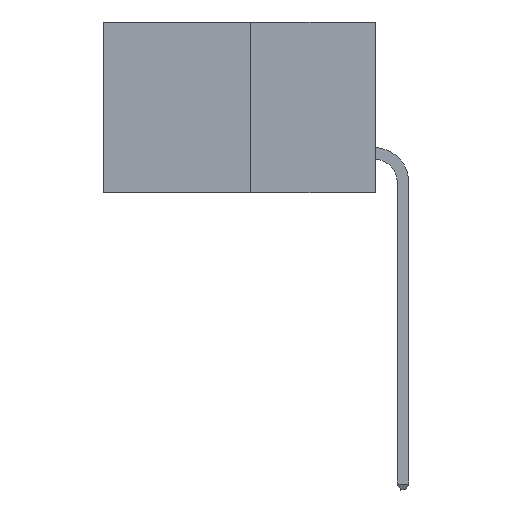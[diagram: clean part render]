
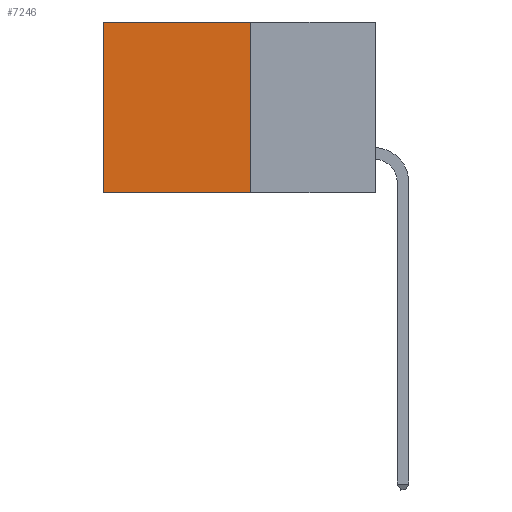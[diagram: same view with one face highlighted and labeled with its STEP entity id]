
A CAD part, left-side view. The second image highlights one B-rep face of the part: STEP entity #7246.
In plain terms, the highlighted planar face has unit normal (-1, 0, 0).
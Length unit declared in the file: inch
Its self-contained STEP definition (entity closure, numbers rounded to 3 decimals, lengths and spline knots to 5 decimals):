
#533 = DIRECTION ( 'NONE',  ( 0., 0., -1. ) ) ;
#584 = DIRECTION ( 'NONE',  ( 1., 0., 0. ) ) ;
#664 = PLANE ( 'NONE',  #7369 ) ;
#1478 = CARTESIAN_POINT ( 'NONE',  ( 0.277, 0.27, -0.37 ) ) ;
#1588 = FACE_OUTER_BOUND ( 'NONE', #15191, .T. ) ;
#1981 = ORIENTED_EDGE ( 'NONE', *, *, #3235, .F. ) ;
#2710 = DIRECTION ( 'NONE',  ( 0., 1., 0. ) ) ;
#2761 = DIRECTION ( 'NONE',  ( 0., 1., 0. ) ) ;
#2790 = CARTESIAN_POINT ( 'NONE',  ( 0.277, 0.27, 0. ) ) ;
#3235 = EDGE_CURVE ( 'NONE', #10393, #20517, #10289, .T. ) ;
#3341 = CARTESIAN_POINT ( 'NONE',  ( 0.277, 0.59, 0. ) ) ;
#4023 = LINE ( 'NONE', #22774, #13128 ) ;
#4284 = CARTESIAN_POINT ( 'NONE',  ( 0.277, 0.27, -0.37 ) ) ;
#4322 = VECTOR ( 'NONE', #2710, 39.37008 ) ;
#4383 = LINE ( 'NONE', #5137, #18283 ) ;
#4416 = ORIENTED_EDGE ( 'NONE', *, *, #5091, .T. ) ;
#4452 = CARTESIAN_POINT ( 'NONE',  ( 0.277, 0.59, -0.37 ) ) ;
#4882 = EDGE_CURVE ( 'NONE', #20253, #21375, #13419, .T. ) ;
#5091 = EDGE_CURVE ( 'NONE', #21375, #20517, #4023, .T. ) ;
#5137 = CARTESIAN_POINT ( 'NONE',  ( 0.277, 0.27, -0.37 ) ) ;
#6927 = DIRECTION ( 'NONE',  ( 0., 0., -1. ) ) ;
#7246 = ADVANCED_FACE ( 'NONE', ( #1588 ), #664, .F. ) ;
#7369 = AXIS2_PLACEMENT_3D ( 'NONE', #1478, #584, #533 ) ;
#10289 = LINE ( 'NONE', #4284, #18812 ) ;
#10393 = VERTEX_POINT ( 'NONE', #15187 ) ;
#11963 = ORIENTED_EDGE ( 'NONE', *, *, #13644, .F. ) ;
#13128 = VECTOR ( 'NONE', #23057, 39.37008 ) ;
#13419 = LINE ( 'NONE', #2790, #4322 ) ;
#13644 = EDGE_CURVE ( 'NONE', #20253, #10393, #4383, .T. ) ;
#15187 = CARTESIAN_POINT ( 'NONE',  ( 0.277, 0.27, -0.37 ) ) ;
#15191 = EDGE_LOOP ( 'NONE', ( #4416, #1981, #11963, #16693 ) ) ;
#16693 = ORIENTED_EDGE ( 'NONE', *, *, #4882, .T. ) ;
#18283 = VECTOR ( 'NONE', #6927, 39.37008 ) ;
#18812 = VECTOR ( 'NONE', #2761, 39.37008 ) ;
#20253 = VERTEX_POINT ( 'NONE', #23174 ) ;
#20517 = VERTEX_POINT ( 'NONE', #4452 ) ;
#21375 = VERTEX_POINT ( 'NONE', #3341 ) ;
#22774 = CARTESIAN_POINT ( 'NONE',  ( 0.277, 0.59, -0.37 ) ) ;
#23057 = DIRECTION ( 'NONE',  ( 0., 0., -1. ) ) ;
#23174 = CARTESIAN_POINT ( 'NONE',  ( 0.277, 0.27, 0. ) ) ;
